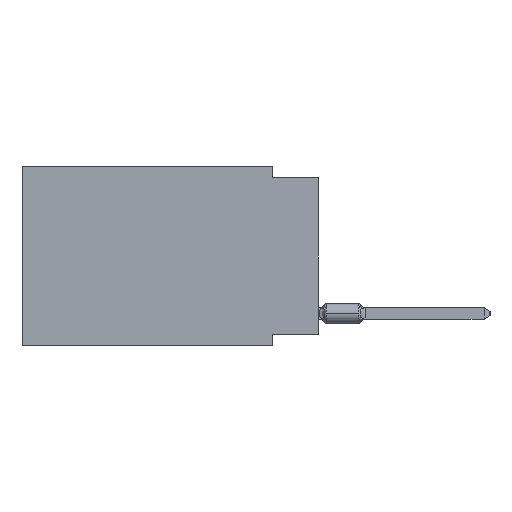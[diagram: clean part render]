
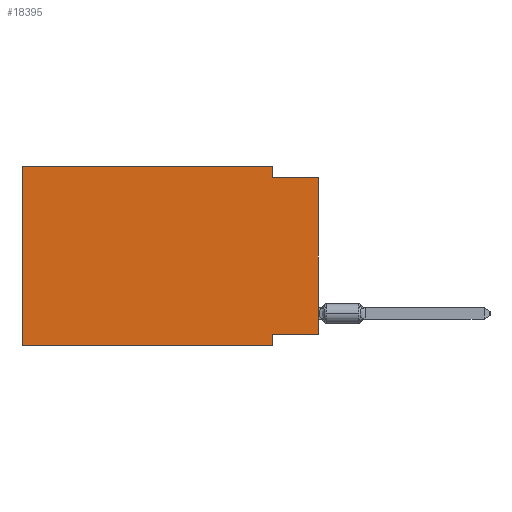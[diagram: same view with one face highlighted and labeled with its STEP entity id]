
A CAD part, left-side view. The second image highlights one B-rep face of the part: STEP entity #18395.
In plain terms, the highlighted planar face has unit normal (-1, 0, 0).
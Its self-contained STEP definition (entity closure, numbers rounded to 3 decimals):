
#969 = DIRECTION ( 'NONE',  ( 0., 1., 0. ) ) ;
#1821 = CARTESIAN_POINT ( 'NONE',  ( 0., 0., 0. ) ) ;
#2565 = CARTESIAN_POINT ( 'NONE',  ( 0., 16.383, 0. ) ) ;
#2889 = CARTESIAN_POINT ( 'NONE',  ( 0., 16.383, 0. ) ) ;
#3621 = CARTESIAN_POINT ( 'NONE',  ( 0., 16.383, 0. ) ) ;
#5807 = EDGE_CURVE ( 'NONE', #71699, #27893, #9959, .T. ) ;
#6488 = EDGE_CURVE ( 'NONE', #35561, #55031, #42158, .T. ) ;
#6583 = DIRECTION ( 'NONE',  ( 0., 0., 1. ) ) ;
#7295 = CARTESIAN_POINT ( 'NONE',  ( 0., 0., -0.635 ) ) ;
#8317 = CARTESIAN_POINT ( 'NONE',  ( 0., 16.383, -9.906 ) ) ;
#9735 = ORIENTED_EDGE ( 'NONE', *, *, #75426, .F. ) ;
#9959 = LINE ( 'NONE', #82073, #20695 ) ;
#10443 = ORIENTED_EDGE ( 'NONE', *, *, #6488, .F. ) ;
#11800 = EDGE_CURVE ( 'NONE', #70592, #24245, #48405, .T. ) ;
#14384 = LINE ( 'NONE', #81301, #79003 ) ;
#15493 = FACE_OUTER_BOUND ( 'NONE', #51805, .T. ) ;
#15727 = VECTOR ( 'NONE', #22884, 1000. ) ;
#16159 = CARTESIAN_POINT ( 'NONE',  ( 0., 2.54, 0. ) ) ;
#17808 = EDGE_CURVE ( 'NONE', #48706, #71699, #27302, .T. ) ;
#17817 = EDGE_CURVE ( 'NONE', #48706, #24245, #80397, .T. ) ;
#18395 = ADVANCED_FACE ( 'NONE', ( #15493 ), #61307, .F. ) ;
#20695 = VECTOR ( 'NONE', #49267, 1000. ) ;
#21232 = VECTOR ( 'NONE', #6583, 1000. ) ;
#22059 = CARTESIAN_POINT ( 'NONE',  ( 0., 0., -0.635 ) ) ;
#22884 = DIRECTION ( 'NONE',  ( 0., -1., 0. ) ) ;
#24245 = VERTEX_POINT ( 'NONE', #7295 ) ;
#24585 = ORIENTED_EDGE ( 'NONE', *, *, #5807, .F. ) ;
#25904 = LINE ( 'NONE', #52248, #43351 ) ;
#27302 = LINE ( 'NONE', #67475, #29496 ) ;
#27893 = VERTEX_POINT ( 'NONE', #35070 ) ;
#28149 = CARTESIAN_POINT ( 'NONE',  ( 0., 16.383, 0. ) ) ;
#29496 = VECTOR ( 'NONE', #969, 1000. ) ;
#31374 = ORIENTED_EDGE ( 'NONE', *, *, #17817, .T. ) ;
#34668 = DIRECTION ( 'NONE',  ( 0., 0., -1. ) ) ;
#35070 = CARTESIAN_POINT ( 'NONE',  ( 0., 2.54, -9.906 ) ) ;
#35561 = VERTEX_POINT ( 'NONE', #8317 ) ;
#42158 = LINE ( 'NONE', #2889, #46776 ) ;
#43351 = VECTOR ( 'NONE', #78601, 1000. ) ;
#46776 = VECTOR ( 'NONE', #81038, 1000. ) ;
#48405 = LINE ( 'NONE', #22059, #15727 ) ;
#48706 = VERTEX_POINT ( 'NONE', #84020 ) ;
#48743 = DIRECTION ( 'NONE',  ( 0., 0., -1. ) ) ;
#48973 = AXIS2_PLACEMENT_3D ( 'NONE', #2565, #81578, #48743 ) ;
#49267 = DIRECTION ( 'NONE',  ( 0., 0., -1. ) ) ;
#49811 = ORIENTED_EDGE ( 'NONE', *, *, #50877, .F. ) ;
#50877 = EDGE_CURVE ( 'NONE', #55031, #68791, #56750, .T. ) ;
#51805 = EDGE_LOOP ( 'NONE', ( #31374, #56165, #9735, #49811, #10443, #84196, #24585, #76325 ) ) ;
#52248 = CARTESIAN_POINT ( 'NONE',  ( 0., 16.383, -9.906 ) ) ;
#55031 = VERTEX_POINT ( 'NONE', #28149 ) ;
#55504 = CARTESIAN_POINT ( 'NONE',  ( 0., 2.54, -0.635 ) ) ;
#56165 = ORIENTED_EDGE ( 'NONE', *, *, #11800, .F. ) ;
#56750 = LINE ( 'NONE', #3621, #60685 ) ;
#60685 = VECTOR ( 'NONE', #76164, 1000. ) ;
#61307 = PLANE ( 'NONE',  #48973 ) ;
#67475 = CARTESIAN_POINT ( 'NONE',  ( 0., 0., -9.271 ) ) ;
#68791 = VERTEX_POINT ( 'NONE', #16159 ) ;
#70592 = VERTEX_POINT ( 'NONE', #55504 ) ;
#71699 = VERTEX_POINT ( 'NONE', #76628 ) ;
#75426 = EDGE_CURVE ( 'NONE', #68791, #70592, #14384, .T. ) ;
#76164 = DIRECTION ( 'NONE',  ( 0., -1., 0. ) ) ;
#76325 = ORIENTED_EDGE ( 'NONE', *, *, #17808, .F. ) ;
#76628 = CARTESIAN_POINT ( 'NONE',  ( 0., 2.54, -9.271 ) ) ;
#77804 = EDGE_CURVE ( 'NONE', #35561, #27893, #25904, .T. ) ;
#78601 = DIRECTION ( 'NONE',  ( 0., -1., 0. ) ) ;
#79003 = VECTOR ( 'NONE', #34668, 1000. ) ;
#80397 = LINE ( 'NONE', #1821, #21232 ) ;
#81038 = DIRECTION ( 'NONE',  ( 0., 0., 1. ) ) ;
#81301 = CARTESIAN_POINT ( 'NONE',  ( 0., 2.54, 0. ) ) ;
#81578 = DIRECTION ( 'NONE',  ( 1., 0., 0. ) ) ;
#82073 = CARTESIAN_POINT ( 'NONE',  ( 0., 2.54, -9.906 ) ) ;
#84020 = CARTESIAN_POINT ( 'NONE',  ( 0., 0., -9.271 ) ) ;
#84196 = ORIENTED_EDGE ( 'NONE', *, *, #77804, .T. ) ;
